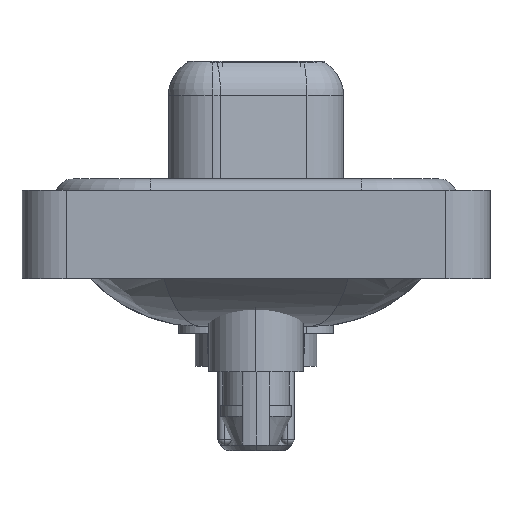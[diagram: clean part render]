
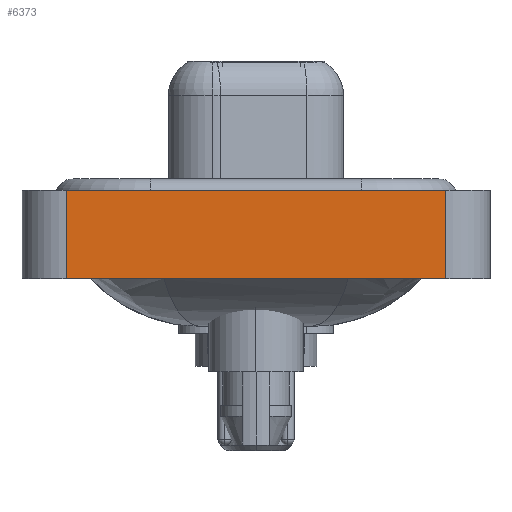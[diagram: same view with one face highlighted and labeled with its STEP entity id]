
A CAD part, left-side view. The second image highlights one B-rep face of the part: STEP entity #6373.
In plain terms, the highlighted planar face has unit normal (-1, 0, 0).
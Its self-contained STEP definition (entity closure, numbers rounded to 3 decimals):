
#47 = EDGE_CURVE ( 'NONE', #20612, #24230, #22142, .T. ) ;
#896 = DIRECTION ( 'NONE',  ( 0., 0., 1. ) ) ;
#1571 = CARTESIAN_POINT ( 'NONE',  ( -7.35, -8.55, 0.4 ) ) ;
#2052 = AXIS2_PLACEMENT_3D ( 'NONE', #8183, #22797, #24962 ) ;
#4126 = LINE ( 'NONE', #4370, #14973 ) ;
#4370 = CARTESIAN_POINT ( 'NONE',  ( -7.35, -8.55, -3.6 ) ) ;
#5474 = VECTOR ( 'NONE', #11603, 1000. ) ;
#6373 = ADVANCED_FACE ( 'NONE', ( #16628 ), #22936, .T. ) ;
#7085 = ORIENTED_EDGE ( 'NONE', *, *, #20666, .F. ) ;
#7848 = VERTEX_POINT ( 'NONE', #15867 ) ;
#8183 = CARTESIAN_POINT ( 'NONE',  ( -7.35, -8.55, -3.6 ) ) ;
#9499 = EDGE_LOOP ( 'NONE', ( #14033, #15768, #7085, #24999 ) ) ;
#10884 = CARTESIAN_POINT ( 'NONE',  ( -7.35, -8.55, -3.6 ) ) ;
#11603 = DIRECTION ( 'NONE',  ( 0., 0., 1. ) ) ;
#13208 = CARTESIAN_POINT ( 'NONE',  ( -7.35, 8.55, 0.4 ) ) ;
#13674 = CARTESIAN_POINT ( 'NONE',  ( -7.35, -8.55, 0.4 ) ) ;
#14033 = ORIENTED_EDGE ( 'NONE', *, *, #47, .T. ) ;
#14243 = VERTEX_POINT ( 'NONE', #13208 ) ;
#14519 = DIRECTION ( 'NONE',  ( 0., -1., 0. ) ) ;
#14973 = VECTOR ( 'NONE', #25159, 1000. ) ;
#15768 = ORIENTED_EDGE ( 'NONE', *, *, #24759, .F. ) ;
#15867 = CARTESIAN_POINT ( 'NONE',  ( -7.35, 8.55, -3.6 ) ) ;
#16628 = FACE_OUTER_BOUND ( 'NONE', #9499, .T. ) ;
#16681 = VECTOR ( 'NONE', #14519, 1000. ) ;
#18955 = VECTOR ( 'NONE', #896, 1000. ) ;
#20054 = LINE ( 'NONE', #24399, #18955 ) ;
#20612 = VERTEX_POINT ( 'NONE', #10884 ) ;
#20666 = EDGE_CURVE ( 'NONE', #7848, #14243, #20054, .T. ) ;
#20712 = LINE ( 'NONE', #1571, #16681 ) ;
#22142 = LINE ( 'NONE', #24024, #5474 ) ;
#22797 = DIRECTION ( 'NONE',  ( -1., 0., 0. ) ) ;
#22936 = PLANE ( 'NONE',  #2052 ) ;
#24024 = CARTESIAN_POINT ( 'NONE',  ( -7.35, -8.55, -3.6 ) ) ;
#24230 = VERTEX_POINT ( 'NONE', #13674 ) ;
#24399 = CARTESIAN_POINT ( 'NONE',  ( -7.35, 8.55, -3.6 ) ) ;
#24759 = EDGE_CURVE ( 'NONE', #14243, #24230, #20712, .T. ) ;
#24962 = DIRECTION ( 'NONE',  ( 0., 0., 1. ) ) ;
#24999 = ORIENTED_EDGE ( 'NONE', *, *, #25191, .T. ) ;
#25159 = DIRECTION ( 'NONE',  ( 0., -1., 0. ) ) ;
#25191 = EDGE_CURVE ( 'NONE', #7848, #20612, #4126, .T. ) ;
